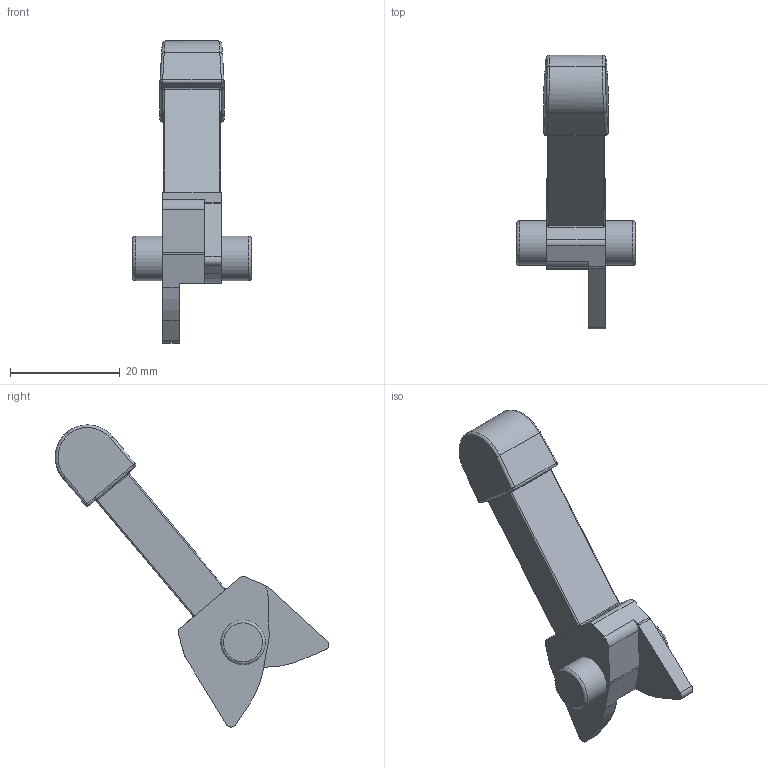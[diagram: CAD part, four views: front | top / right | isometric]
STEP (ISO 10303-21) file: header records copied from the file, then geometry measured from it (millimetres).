
FILE_DESCRIPTION(/* description */ (''),/* implementation_level */ '2;1');
FILE_NAME(/* name */ 'freeloader-lever-v3.step',/* time_stamp */ '2021-09-20T14:44:21-07:00',/* author */ (''),/* organization */ (''),/* preprocessor_version */ 'ST-DEVELOPER v18.1',/* originating_system */ 'Autodesk Translation Framework v10.10.0.1391',/* authorisation */ '');
FILE_SCHEMA (('AUTOMOTIVE_DESIGN { 1 0 10303 214 3 1 1 }'));
Length unit declared in the file: millimetre
Products named in the file (1): loader-lever
Bounding box: 21.71 x 49.86 x 55.09 mm (x, y, z)
Volume: 7019.7 mm3; surface area: 3273.7 mm2
Topology: 1 solids, 1 shells, 87 faces, 208 edges, 126 vertices
Faces by surface type: cylinder 38, plane 27, torus 10, bspline 8, sphere 4
Full cylindrical faces by diameter (mm): 8.12 x2
Entity records: 2813 total; most frequent: CARTESIAN_POINT 742, DIRECTION 448, ORIENTED_EDGE 416, EDGE_CURVE 208, AXIS2_PLACEMENT_3D 174, VERTEX_POINT 126, LINE 100, VECTOR 100
